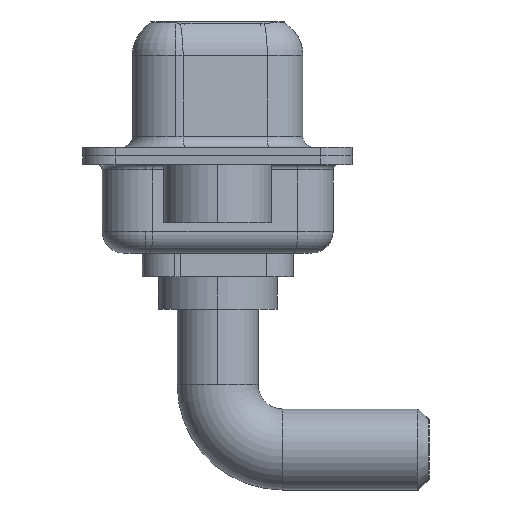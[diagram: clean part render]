
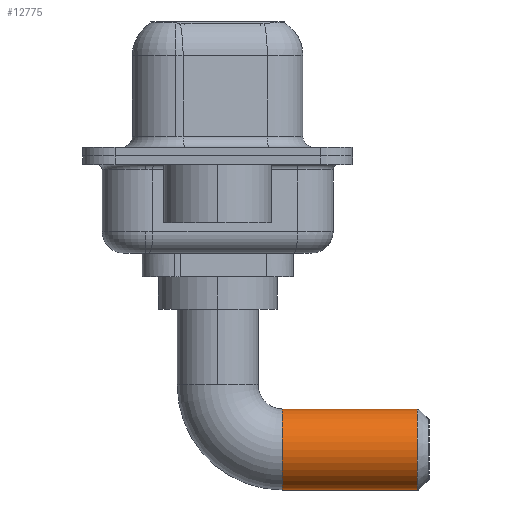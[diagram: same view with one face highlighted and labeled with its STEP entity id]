
A CAD part, left-side view. The second image highlights one B-rep face of the part: STEP entity #12775.
In plain terms, the highlighted cylindrical face has radius 1.875 mm (diameter 3.75 mm), a partial arc.
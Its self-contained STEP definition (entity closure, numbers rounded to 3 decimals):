
#260 = DIRECTION ( 'NONE',  ( 0., -1., 0. ) ) ;
#304 = CIRCLE ( 'NONE', #5681, 1.875 ) ;
#348 = DIRECTION ( 'NONE',  ( -1., 0., 0. ) ) ;
#1384 = DIRECTION ( 'NONE',  ( 0., 0., -1. ) ) ;
#1655 = CARTESIAN_POINT ( 'NONE',  ( 0., -3., -4.625 ) ) ;
#2654 = CARTESIAN_POINT ( 'NONE',  ( 0., -3., -8.375 ) ) ;
#2671 = ORIENTED_EDGE ( 'NONE', *, *, #5730, .F. ) ;
#3414 = LINE ( 'NONE', #8329, #13130 ) ;
#3779 = CARTESIAN_POINT ( 'NONE',  ( 0., -3., -8.375 ) ) ;
#4928 = DIRECTION ( 'NONE',  ( 0., -1., 0. ) ) ;
#5065 = ORIENTED_EDGE ( 'NONE', *, *, #8034, .T. ) ;
#5212 = CARTESIAN_POINT ( 'NONE',  ( 0., -9.25, -6.5 ) ) ;
#5289 = VERTEX_POINT ( 'NONE', #1655 ) ;
#5681 = AXIS2_PLACEMENT_3D ( 'NONE', #5212, #10314, #1384 ) ;
#5712 = CYLINDRICAL_SURFACE ( 'NONE', #13052, 1.875 ) ;
#5730 = EDGE_CURVE ( 'NONE', #5289, #6930, #3414, .T. ) ;
#6624 = CARTESIAN_POINT ( 'NONE',  ( 0., -9.25, -4.625 ) ) ;
#6766 = VERTEX_POINT ( 'NONE', #2654 ) ;
#6930 = VERTEX_POINT ( 'NONE', #6624 ) ;
#6979 = EDGE_CURVE ( 'NONE', #6766, #7023, #7096, .T. ) ;
#6990 = AXIS2_PLACEMENT_3D ( 'NONE', #9824, #12776, #348 ) ;
#7023 = VERTEX_POINT ( 'NONE', #11914 ) ;
#7096 = LINE ( 'NONE', #3779, #11007 ) ;
#7920 = FACE_OUTER_BOUND ( 'NONE', #11707, .T. ) ;
#8034 = EDGE_CURVE ( 'NONE', #7023, #6930, #304, .T. ) ;
#8329 = CARTESIAN_POINT ( 'NONE',  ( 0., -3., -4.625 ) ) ;
#8662 = EDGE_CURVE ( 'NONE', #5289, #6766, #12324, .T. ) ;
#8731 = DIRECTION ( 'NONE',  ( 0., -1., 0. ) ) ;
#9824 = CARTESIAN_POINT ( 'NONE',  ( 0., -3., -6.5 ) ) ;
#10314 = DIRECTION ( 'NONE',  ( 0., 1., 0. ) ) ;
#10868 = DIRECTION ( 'NONE',  ( 0., 0., -1. ) ) ;
#10934 = CARTESIAN_POINT ( 'NONE',  ( 0., -3., -6.5 ) ) ;
#11007 = VECTOR ( 'NONE', #4928, 1000. ) ;
#11585 = ORIENTED_EDGE ( 'NONE', *, *, #6979, .T. ) ;
#11707 = EDGE_LOOP ( 'NONE', ( #2671, #12777, #11585, #5065 ) ) ;
#11914 = CARTESIAN_POINT ( 'NONE',  ( 0., -9.25, -8.375 ) ) ;
#12324 = CIRCLE ( 'NONE', #6990, 1.875 ) ;
#12775 = ADVANCED_FACE ( 'NONE', ( #7920 ), #5712, .T. ) ;
#12776 = DIRECTION ( 'NONE',  ( 0., -1., 0. ) ) ;
#12777 = ORIENTED_EDGE ( 'NONE', *, *, #8662, .T. ) ;
#13052 = AXIS2_PLACEMENT_3D ( 'NONE', #10934, #8731, #10868 ) ;
#13130 = VECTOR ( 'NONE', #260, 1000. ) ;
